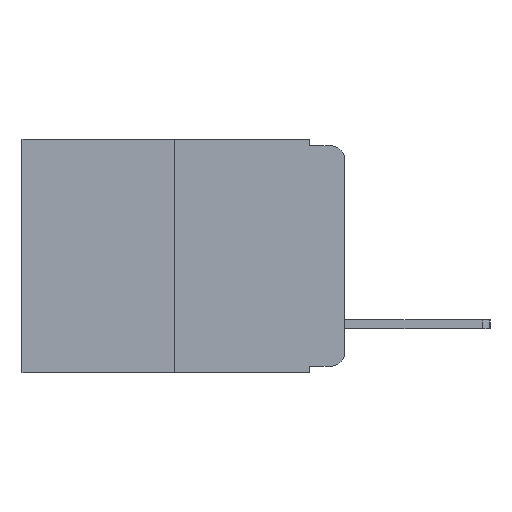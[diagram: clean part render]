
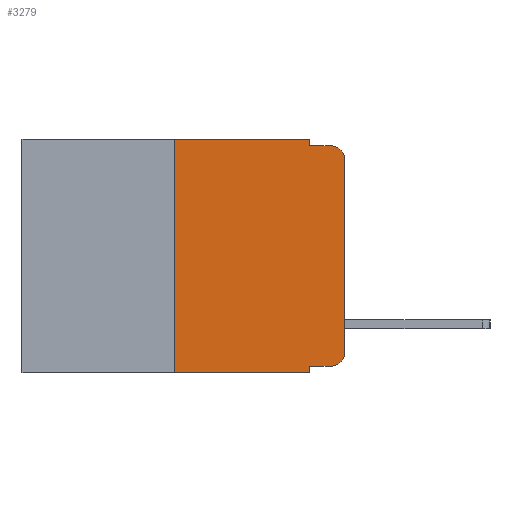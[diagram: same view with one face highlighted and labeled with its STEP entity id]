
A CAD part, left-side view. The second image highlights one B-rep face of the part: STEP entity #3279.
In plain terms, the highlighted planar face has unit normal (-1, 0, 0).
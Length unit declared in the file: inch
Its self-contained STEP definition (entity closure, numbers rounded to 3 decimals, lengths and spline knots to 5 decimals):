
#441 = ORIENTED_EDGE ( 'NONE', *, *, #1012, .T. ) ;
#819 = CARTESIAN_POINT ( 'NONE',  ( 0., 0.02, -0.313 ) ) ;
#907 = DIRECTION ( 'NONE',  ( 0., 0., -1. ) ) ;
#1012 = EDGE_CURVE ( 'NONE', #11511, #13389, #4672, .T. ) ;
#1040 = DIRECTION ( 'NONE',  ( 0., 0., -1. ) ) ;
#1487 = ORIENTED_EDGE ( 'NONE', *, *, #5596, .T. ) ;
#1770 = DIRECTION ( 'NONE',  ( 1., 0., 0. ) ) ;
#1944 = DIRECTION ( 'NONE',  ( 0., -1., 0. ) ) ;
#2097 = LINE ( 'NONE', #15608, #10928 ) ;
#2880 = ORIENTED_EDGE ( 'NONE', *, *, #14322, .F. ) ;
#3046 = ORIENTED_EDGE ( 'NONE', *, *, #17407, .T. ) ;
#3075 = VERTEX_POINT ( 'NONE', #18296 ) ;
#3279 = ADVANCED_FACE ( 'NONE', ( #18015 ), #15724, .F. ) ;
#3426 = VECTOR ( 'NONE', #15797, 39.37008 ) ;
#3482 = EDGE_CURVE ( 'NONE', #20183, #11511, #16736, .T. ) ;
#3613 = CARTESIAN_POINT ( 'NONE',  ( 0., 0.051, -0.333 ) ) ;
#3951 = VERTEX_POINT ( 'NONE', #12335 ) ;
#4017 = VECTOR ( 'NONE', #1944, 39.37008 ) ;
#4077 = AXIS2_PLACEMENT_3D ( 'NONE', #819, #12333, #1040 ) ;
#4672 = CIRCLE ( 'NONE', #4077, 0.02 ) ;
#4690 = EDGE_CURVE ( 'NONE', #20183, #21666, #10762, .T. ) ;
#4734 = VECTOR ( 'NONE', #5172, 39.37008 ) ;
#4812 = ORIENTED_EDGE ( 'NONE', *, *, #11731, .F. ) ;
#4981 = VERTEX_POINT ( 'NONE', #17473 ) ;
#5042 = ORIENTED_EDGE ( 'NONE', *, *, #4690, .F. ) ;
#5172 = DIRECTION ( 'NONE',  ( 0., 0., -1. ) ) ;
#5196 = DIRECTION ( 'NONE',  ( 0., -1., 0. ) ) ;
#5262 = ORIENTED_EDGE ( 'NONE', *, *, #3482, .T. ) ;
#5433 = CARTESIAN_POINT ( 'NONE',  ( 0., 0.473, 0. ) ) ;
#5496 = AXIS2_PLACEMENT_3D ( 'NONE', #18387, #8131, #20033 ) ;
#5596 = EDGE_CURVE ( 'NONE', #4981, #21666, #17271, .T. ) ;
#5849 = EDGE_CURVE ( 'NONE', #4981, #3951, #8366, .T. ) ;
#6033 = CARTESIAN_POINT ( 'NONE',  ( 0., 0.02, -0.333 ) ) ;
#6726 = CIRCLE ( 'NONE', #5496, 0.02 ) ;
#7731 = ORIENTED_EDGE ( 'NONE', *, *, #10534, .F. ) ;
#7984 = CARTESIAN_POINT ( 'NONE',  ( 0., 0.051, 0. ) ) ;
#8131 = DIRECTION ( 'NONE',  ( -1., 0., 0. ) ) ;
#8366 = LINE ( 'NONE', #9662, #17524 ) ;
#8395 = CARTESIAN_POINT ( 'NONE',  ( 0., 0., 0. ) ) ;
#8585 = CARTESIAN_POINT ( 'NONE',  ( 0., 0., -0.03 ) ) ;
#9108 = CARTESIAN_POINT ( 'NONE',  ( 0., 0.473, -0.343 ) ) ;
#9162 = VECTOR ( 'NONE', #17492, 39.37008 ) ;
#9272 = CARTESIAN_POINT ( 'NONE',  ( 0., 0., -0.313 ) ) ;
#9662 = CARTESIAN_POINT ( 'NONE',  ( 0., 0.25, 0. ) ) ;
#10518 = VERTEX_POINT ( 'NONE', #8585 ) ;
#10534 = EDGE_CURVE ( 'NONE', #3075, #16314, #14494, .T. ) ;
#10762 = LINE ( 'NONE', #7984, #14785 ) ;
#10928 = VECTOR ( 'NONE', #5196, 39.37008 ) ;
#11425 = DIRECTION ( 'NONE',  ( 0., 0., 1. ) ) ;
#11511 = VERTEX_POINT ( 'NONE', #6033 ) ;
#11731 = EDGE_CURVE ( 'NONE', #16314, #14216, #2097, .T. ) ;
#11744 = ORIENTED_EDGE ( 'NONE', *, *, #5849, .F. ) ;
#11770 = CARTESIAN_POINT ( 'NONE',  ( 0., 0.051, -0.343 ) ) ;
#11775 = AXIS2_PLACEMENT_3D ( 'NONE', #12354, #1770, #14022 ) ;
#12333 = DIRECTION ( 'NONE',  ( -1., 0., 0. ) ) ;
#12335 = CARTESIAN_POINT ( 'NONE',  ( 0., 0.25, 0. ) ) ;
#12354 = CARTESIAN_POINT ( 'NONE',  ( 0., 0.473, 0. ) ) ;
#12859 = EDGE_CURVE ( 'NONE', #10518, #14216, #6726, .T. ) ;
#13389 = VERTEX_POINT ( 'NONE', #9272 ) ;
#13778 = LINE ( 'NONE', #5433, #9162 ) ;
#14022 = DIRECTION ( 'NONE',  ( 0., 0., -1. ) ) ;
#14186 = VECTOR ( 'NONE', #20266, 39.37008 ) ;
#14216 = VERTEX_POINT ( 'NONE', #15475 ) ;
#14322 = EDGE_CURVE ( 'NONE', #3951, #3075, #13778, .T. ) ;
#14494 = LINE ( 'NONE', #18879, #4734 ) ;
#14785 = VECTOR ( 'NONE', #907, 39.37008 ) ;
#14800 = CARTESIAN_POINT ( 'NONE',  ( 0., 0.051, -0.01 ) ) ;
#15475 = CARTESIAN_POINT ( 'NONE',  ( 0., 0.02, -0.01 ) ) ;
#15608 = CARTESIAN_POINT ( 'NONE',  ( 0., 0.051, -0.01 ) ) ;
#15724 = PLANE ( 'NONE',  #11775 ) ;
#15797 = DIRECTION ( 'NONE',  ( 0., -1., 0. ) ) ;
#16314 = VERTEX_POINT ( 'NONE', #14800 ) ;
#16736 = LINE ( 'NONE', #3613, #3426 ) ;
#16815 = EDGE_LOOP ( 'NONE', ( #3046, #18527, #4812, #7731, #2880, #11744, #1487, #5042, #5262, #441 ) ) ;
#17271 = LINE ( 'NONE', #9108, #4017 ) ;
#17407 = EDGE_CURVE ( 'NONE', #13389, #10518, #19158, .T. ) ;
#17473 = CARTESIAN_POINT ( 'NONE',  ( 0., 0.25, -0.343 ) ) ;
#17492 = DIRECTION ( 'NONE',  ( 0., -1., 0. ) ) ;
#17524 = VECTOR ( 'NONE', #11425, 39.37008 ) ;
#18015 = FACE_OUTER_BOUND ( 'NONE', #16815, .T. ) ;
#18296 = CARTESIAN_POINT ( 'NONE',  ( 0., 0.051, 0. ) ) ;
#18387 = CARTESIAN_POINT ( 'NONE',  ( 0., 0.02, -0.03 ) ) ;
#18527 = ORIENTED_EDGE ( 'NONE', *, *, #12859, .T. ) ;
#18879 = CARTESIAN_POINT ( 'NONE',  ( 0., 0.051, 0. ) ) ;
#19158 = LINE ( 'NONE', #8395, #14186 ) ;
#20033 = DIRECTION ( 'NONE',  ( 0., 0., -1. ) ) ;
#20183 = VERTEX_POINT ( 'NONE', #22150 ) ;
#20266 = DIRECTION ( 'NONE',  ( 0., 0., 1. ) ) ;
#21666 = VERTEX_POINT ( 'NONE', #11770 ) ;
#22150 = CARTESIAN_POINT ( 'NONE',  ( 0., 0.051, -0.333 ) ) ;
